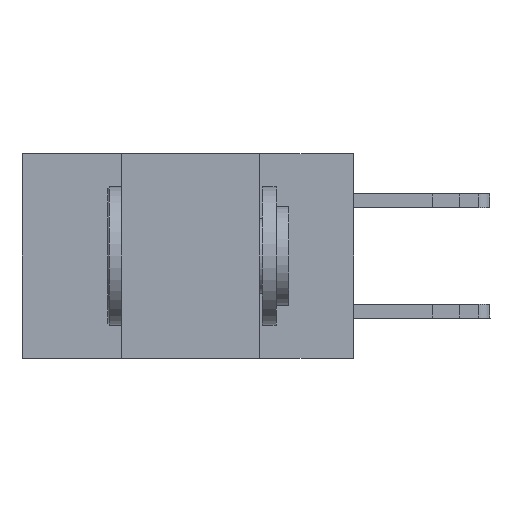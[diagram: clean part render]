
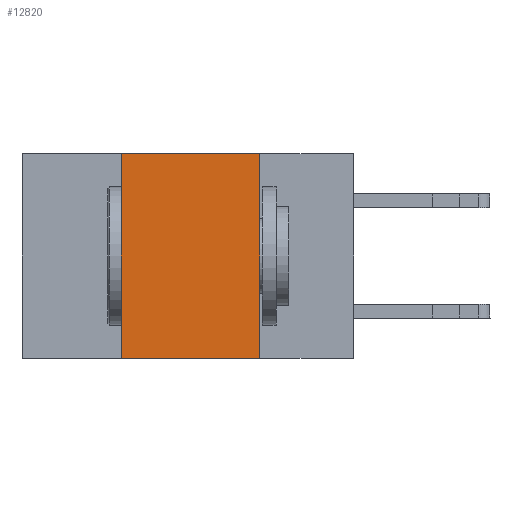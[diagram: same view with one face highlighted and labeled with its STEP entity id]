
A CAD part, left-side view. The second image highlights one B-rep face of the part: STEP entity #12820.
In plain terms, the highlighted planar face has unit normal (-1, 0, 0).
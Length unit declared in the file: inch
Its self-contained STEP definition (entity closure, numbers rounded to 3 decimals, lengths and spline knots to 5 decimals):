
#398 = CARTESIAN_POINT ( 'NONE',  ( 0., 0.17, -0.37 ) ) ;
#430 = EDGE_CURVE ( 'NONE', #11022, #8093, #9012, .T. ) ;
#1021 = CARTESIAN_POINT ( 'NONE',  ( 0., 0.6, 0. ) ) ;
#1169 = VECTOR ( 'NONE', #13966, 39.37008 ) ;
#1549 = CARTESIAN_POINT ( 'NONE',  ( 0., 0.6, 0. ) ) ;
#1730 = EDGE_CURVE ( 'NONE', #1982, #8093, #7473, .T. ) ;
#1982 = VERTEX_POINT ( 'NONE', #7203 ) ;
#3664 = LINE ( 'NONE', #1021, #15382 ) ;
#3857 = ORIENTED_EDGE ( 'NONE', *, *, #430, .F. ) ;
#3907 = CARTESIAN_POINT ( 'NONE',  ( 0., 0.6, -0.37 ) ) ;
#4102 = DIRECTION ( 'NONE',  ( 0., 0., -1. ) ) ;
#5617 = ORIENTED_EDGE ( 'NONE', *, *, #9766, .F. ) ;
#6112 = ORIENTED_EDGE ( 'NONE', *, *, #13201, .F. ) ;
#7203 = CARTESIAN_POINT ( 'NONE',  ( 0., 0.42, -0.37 ) ) ;
#7298 = DIRECTION ( 'NONE',  ( 0., -1., 0. ) ) ;
#7473 = LINE ( 'NONE', #3907, #1169 ) ;
#7976 = DIRECTION ( 'NONE',  ( 0., 0., -1. ) ) ;
#7998 = AXIS2_PLACEMENT_3D ( 'NONE', #1549, #8021, #4102 ) ;
#8021 = DIRECTION ( 'NONE',  ( 1., 0., 0. ) ) ;
#8093 = VERTEX_POINT ( 'NONE', #398 ) ;
#8411 = CARTESIAN_POINT ( 'NONE',  ( 0., 0.42, 0. ) ) ;
#8856 = VECTOR ( 'NONE', #14665, 39.37008 ) ;
#8893 = ORIENTED_EDGE ( 'NONE', *, *, #1730, .T. ) ;
#9012 = LINE ( 'NONE', #11741, #16671 ) ;
#9485 = FACE_OUTER_BOUND ( 'NONE', #14061, .T. ) ;
#9743 = CARTESIAN_POINT ( 'NONE',  ( 0., 0.42, 0. ) ) ;
#9766 = EDGE_CURVE ( 'NONE', #11772, #11022, #3664, .T. ) ;
#11022 = VERTEX_POINT ( 'NONE', #13219 ) ;
#11741 = CARTESIAN_POINT ( 'NONE',  ( 0., 0.17, 0. ) ) ;
#11772 = VERTEX_POINT ( 'NONE', #8411 ) ;
#12820 = ADVANCED_FACE ( 'NONE', ( #9485 ), #14393, .F. ) ;
#13201 = EDGE_CURVE ( 'NONE', #1982, #11772, #16249, .T. ) ;
#13219 = CARTESIAN_POINT ( 'NONE',  ( 0., 0.17, 0. ) ) ;
#13966 = DIRECTION ( 'NONE',  ( 0., -1., 0. ) ) ;
#14061 = EDGE_LOOP ( 'NONE', ( #3857, #5617, #6112, #8893 ) ) ;
#14393 = PLANE ( 'NONE',  #7998 ) ;
#14665 = DIRECTION ( 'NONE',  ( 0., 0., 1. ) ) ;
#15382 = VECTOR ( 'NONE', #7298, 39.37008 ) ;
#16249 = LINE ( 'NONE', #9743, #8856 ) ;
#16671 = VECTOR ( 'NONE', #7976, 39.37008 ) ;
